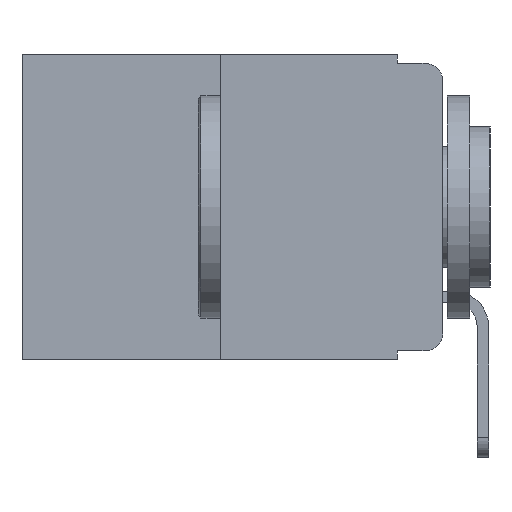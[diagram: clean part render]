
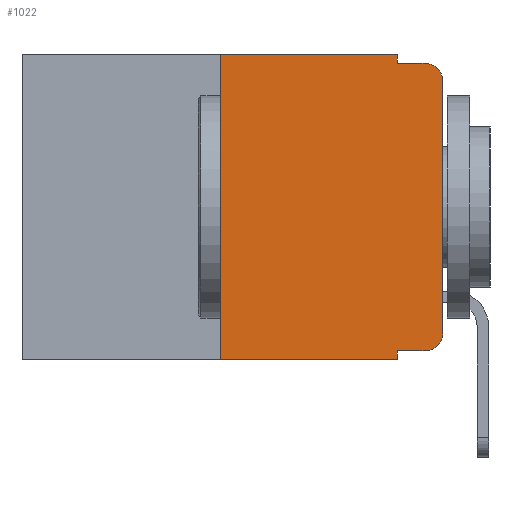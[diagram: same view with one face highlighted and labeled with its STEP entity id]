
A CAD part, left-side view. The second image highlights one B-rep face of the part: STEP entity #1022.
In plain terms, the highlighted planar face has unit normal (-1, 0, 0).
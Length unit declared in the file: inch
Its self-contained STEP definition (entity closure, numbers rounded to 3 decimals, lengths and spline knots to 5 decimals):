
#146 = EDGE_CURVE ( 'NONE', #7066, #13434, #1873, .T. ) ;
#178 = VECTOR ( 'NONE', #11810, 39.37008 ) ;
#309 = ORIENTED_EDGE ( 'NONE', *, *, #10961, .T. ) ;
#392 = DIRECTION ( 'NONE',  ( 0., 0., -1. ) ) ;
#406 = DIRECTION ( 'NONE',  ( 0., -1., 0. ) ) ;
#507 = VECTOR ( 'NONE', #11985, 39.37008 ) ;
#704 = EDGE_CURVE ( 'NONE', #13434, #1655, #10429, .T. ) ;
#899 = LINE ( 'NONE', #2915, #507 ) ;
#1022 = ADVANCED_FACE ( 'NONE', ( #9082 ), #7925, .F. ) ;
#1033 = EDGE_CURVE ( 'NONE', #1267, #1655, #3975, .T. ) ;
#1076 = DIRECTION ( 'NONE',  ( 0., 0., 1. ) ) ;
#1107 = CARTESIAN_POINT ( 'NONE',  ( 0., 0.473, -0.343 ) ) ;
#1267 = VERTEX_POINT ( 'NONE', #8123 ) ;
#1463 = CARTESIAN_POINT ( 'NONE',  ( 0., 0.051, -0.333 ) ) ;
#1583 = CARTESIAN_POINT ( 'NONE',  ( 0., 0.473, 0. ) ) ;
#1637 = CARTESIAN_POINT ( 'NONE',  ( 0., 0.25, 0. ) ) ;
#1655 = VERTEX_POINT ( 'NONE', #6141 ) ;
#1817 = ORIENTED_EDGE ( 'NONE', *, *, #2238, .T. ) ;
#1854 = CARTESIAN_POINT ( 'NONE',  ( 0., 0.02, -0.313 ) ) ;
#1873 = LINE ( 'NONE', #5657, #11837 ) ;
#1943 = DIRECTION ( 'NONE',  ( -1., 0., 0. ) ) ;
#2216 = VECTOR ( 'NONE', #10488, 39.37008 ) ;
#2238 = EDGE_CURVE ( 'NONE', #9603, #1267, #3931, .T. ) ;
#2298 = DIRECTION ( 'NONE',  ( 0., -1., 0. ) ) ;
#2835 = EDGE_CURVE ( 'NONE', #12569, #9603, #8122, .T. ) ;
#2871 = CARTESIAN_POINT ( 'NONE',  ( 0., 0., -0.313 ) ) ;
#2906 = ORIENTED_EDGE ( 'NONE', *, *, #10552, .F. ) ;
#2915 = CARTESIAN_POINT ( 'NONE',  ( 0., 0.051, 0. ) ) ;
#3308 = DIRECTION ( 'NONE',  ( 0., 0., -1. ) ) ;
#3332 = LINE ( 'NONE', #1463, #178 ) ;
#3818 = CARTESIAN_POINT ( 'NONE',  ( 0., 0.051, 0. ) ) ;
#3931 = LINE ( 'NONE', #8746, #6125 ) ;
#3975 = CIRCLE ( 'NONE', #8376, 0.02 ) ;
#3995 = CARTESIAN_POINT ( 'NONE',  ( 0., 0.051, -0.01 ) ) ;
#4636 = ORIENTED_EDGE ( 'NONE', *, *, #2835, .T. ) ;
#4946 = ORIENTED_EDGE ( 'NONE', *, *, #704, .F. ) ;
#5054 = VERTEX_POINT ( 'NONE', #13090 ) ;
#5657 = CARTESIAN_POINT ( 'NONE',  ( 0., 0.051, 0. ) ) ;
#5772 = EDGE_LOOP ( 'NONE', ( #1817, #11337, #4946, #7271, #2906, #7736, #309, #9851, #6176, #4636 ) ) ;
#5854 = CARTESIAN_POINT ( 'NONE',  ( 0., 0.051, -0.343 ) ) ;
#6125 = VECTOR ( 'NONE', #6959, 39.37008 ) ;
#6141 = CARTESIAN_POINT ( 'NONE',  ( 0., 0.02, -0.01 ) ) ;
#6176 = ORIENTED_EDGE ( 'NONE', *, *, #12351, .T. ) ;
#6316 = VERTEX_POINT ( 'NONE', #9793 ) ;
#6321 = VERTEX_POINT ( 'NONE', #5854 ) ;
#6546 = LINE ( 'NONE', #8601, #11079 ) ;
#6959 = DIRECTION ( 'NONE',  ( 0., 0., 1. ) ) ;
#7026 = CARTESIAN_POINT ( 'NONE',  ( 0., 0.02, -0.03 ) ) ;
#7066 = VERTEX_POINT ( 'NONE', #3818 ) ;
#7271 = ORIENTED_EDGE ( 'NONE', *, *, #146, .F. ) ;
#7736 = ORIENTED_EDGE ( 'NONE', *, *, #12760, .F. ) ;
#7918 = CARTESIAN_POINT ( 'NONE',  ( 0., 0.473, 0. ) ) ;
#7925 = PLANE ( 'NONE',  #9006 ) ;
#8007 = DIRECTION ( 'NONE',  ( 0., 0., -1. ) ) ;
#8046 = DIRECTION ( 'NONE',  ( 1., 0., 0. ) ) ;
#8122 = CIRCLE ( 'NONE', #8137, 0.02 ) ;
#8123 = CARTESIAN_POINT ( 'NONE',  ( 0., 0., -0.03 ) ) ;
#8137 = AXIS2_PLACEMENT_3D ( 'NONE', #1854, #1943, #3308 ) ;
#8376 = AXIS2_PLACEMENT_3D ( 'NONE', #7026, #13424, #13094 ) ;
#8433 = LINE ( 'NONE', #1107, #13222 ) ;
#8439 = CARTESIAN_POINT ( 'NONE',  ( 0., 0.051, -0.01 ) ) ;
#8601 = CARTESIAN_POINT ( 'NONE',  ( 0., 0.25, 0. ) ) ;
#8746 = CARTESIAN_POINT ( 'NONE',  ( 0., 0., 0. ) ) ;
#9006 = AXIS2_PLACEMENT_3D ( 'NONE', #7918, #8046, #8007 ) ;
#9082 = FACE_OUTER_BOUND ( 'NONE', #5772, .T. ) ;
#9168 = VECTOR ( 'NONE', #406, 39.37008 ) ;
#9603 = VERTEX_POINT ( 'NONE', #2871 ) ;
#9793 = CARTESIAN_POINT ( 'NONE',  ( 0., 0.051, -0.333 ) ) ;
#9851 = ORIENTED_EDGE ( 'NONE', *, *, #13460, .F. ) ;
#10429 = LINE ( 'NONE', #8439, #2216 ) ;
#10488 = DIRECTION ( 'NONE',  ( 0., -1., 0. ) ) ;
#10552 = EDGE_CURVE ( 'NONE', #10586, #7066, #11737, .T. ) ;
#10586 = VERTEX_POINT ( 'NONE', #1637 ) ;
#10961 = EDGE_CURVE ( 'NONE', #5054, #6321, #8433, .T. ) ;
#11079 = VECTOR ( 'NONE', #1076, 39.37008 ) ;
#11337 = ORIENTED_EDGE ( 'NONE', *, *, #1033, .T. ) ;
#11737 = LINE ( 'NONE', #1583, #9168 ) ;
#11810 = DIRECTION ( 'NONE',  ( 0., -1., 0. ) ) ;
#11837 = VECTOR ( 'NONE', #392, 39.37008 ) ;
#11985 = DIRECTION ( 'NONE',  ( 0., 0., -1. ) ) ;
#12079 = CARTESIAN_POINT ( 'NONE',  ( 0., 0.02, -0.333 ) ) ;
#12351 = EDGE_CURVE ( 'NONE', #6316, #12569, #3332, .T. ) ;
#12569 = VERTEX_POINT ( 'NONE', #12079 ) ;
#12760 = EDGE_CURVE ( 'NONE', #5054, #10586, #6546, .T. ) ;
#13090 = CARTESIAN_POINT ( 'NONE',  ( 0., 0.25, -0.343 ) ) ;
#13094 = DIRECTION ( 'NONE',  ( 0., 0., -1. ) ) ;
#13222 = VECTOR ( 'NONE', #2298, 39.37008 ) ;
#13424 = DIRECTION ( 'NONE',  ( -1., 0., 0. ) ) ;
#13434 = VERTEX_POINT ( 'NONE', #3995 ) ;
#13460 = EDGE_CURVE ( 'NONE', #6316, #6321, #899, .T. ) ;
